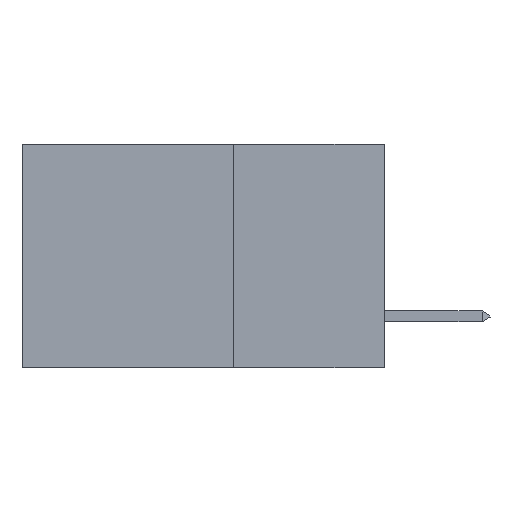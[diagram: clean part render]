
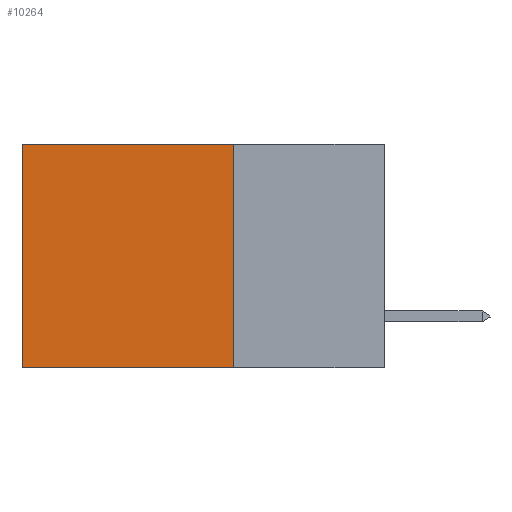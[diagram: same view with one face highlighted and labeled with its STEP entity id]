
A CAD part, left-side view. The second image highlights one B-rep face of the part: STEP entity #10264.
In plain terms, the highlighted planar face has unit normal (-1, 0, 0).
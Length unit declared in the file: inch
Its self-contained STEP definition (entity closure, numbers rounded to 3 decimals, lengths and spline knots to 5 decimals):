
#300 = CARTESIAN_POINT ( 'NONE',  ( 0.2875, 0.25, 0. ) ) ;
#1099 = VERTEX_POINT ( 'NONE', #3515 ) ;
#1140 = LINE ( 'NONE', #6126, #1829 ) ;
#1829 = VECTOR ( 'NONE', #17146, 39.37008 ) ;
#2435 = EDGE_CURVE ( 'NONE', #11167, #4424, #5220, .T. ) ;
#2447 = CARTESIAN_POINT ( 'NONE',  ( 0.2875, 0.25, -0.37 ) ) ;
#3110 = CARTESIAN_POINT ( 'NONE',  ( 0.2875, 0.25, 0. ) ) ;
#3515 = CARTESIAN_POINT ( 'NONE',  ( 0.2875, 0.6, 0. ) ) ;
#3711 = VECTOR ( 'NONE', #9554, 39.37008 ) ;
#4189 = CARTESIAN_POINT ( 'NONE',  ( 0.2875, 0.25, -0.37 ) ) ;
#4190 = VECTOR ( 'NONE', #6963, 39.37008 ) ;
#4424 = VERTEX_POINT ( 'NONE', #2447 ) ;
#4636 = VECTOR ( 'NONE', #16760, 39.37008 ) ;
#5220 = LINE ( 'NONE', #15196, #3711 ) ;
#5274 = FACE_OUTER_BOUND ( 'NONE', #11507, .T. ) ;
#5278 = ORIENTED_EDGE ( 'NONE', *, *, #16095, .F. ) ;
#6126 = CARTESIAN_POINT ( 'NONE',  ( 0.2875, 0.6, 0. ) ) ;
#6963 = DIRECTION ( 'NONE',  ( 0., 1., 0. ) ) ;
#7256 = VERTEX_POINT ( 'NONE', #7313 ) ;
#7297 = DIRECTION ( 'NONE',  ( 0., 0., -1. ) ) ;
#7313 = CARTESIAN_POINT ( 'NONE',  ( 0.2875, 0.6, -0.37 ) ) ;
#8402 = EDGE_CURVE ( 'NONE', #1099, #7256, #1140, .T. ) ;
#9554 = DIRECTION ( 'NONE',  ( 0., 0., -1. ) ) ;
#10019 = ORIENTED_EDGE ( 'NONE', *, *, #2435, .F. ) ;
#10062 = DIRECTION ( 'NONE',  ( 1., 0., 0. ) ) ;
#10264 = ADVANCED_FACE ( 'NONE', ( #5274 ), #11412, .F. ) ;
#11167 = VERTEX_POINT ( 'NONE', #300 ) ;
#11385 = CARTESIAN_POINT ( 'NONE',  ( 0.2875, 0.25, 0. ) ) ;
#11386 = LINE ( 'NONE', #11385, #4190 ) ;
#11412 = PLANE ( 'NONE',  #16078 ) ;
#11507 = EDGE_LOOP ( 'NONE', ( #14045, #5278, #10019, #16907 ) ) ;
#14045 = ORIENTED_EDGE ( 'NONE', *, *, #8402, .T. ) ;
#15196 = CARTESIAN_POINT ( 'NONE',  ( 0.2875, 0.25, 0. ) ) ;
#15967 = LINE ( 'NONE', #4189, #4636 ) ;
#16052 = EDGE_CURVE ( 'NONE', #11167, #1099, #11386, .T. ) ;
#16078 = AXIS2_PLACEMENT_3D ( 'NONE', #3110, #10062, #7297 ) ;
#16095 = EDGE_CURVE ( 'NONE', #4424, #7256, #15967, .T. ) ;
#16760 = DIRECTION ( 'NONE',  ( 0., 1., 0. ) ) ;
#16907 = ORIENTED_EDGE ( 'NONE', *, *, #16052, .T. ) ;
#17146 = DIRECTION ( 'NONE',  ( 0., 0., -1. ) ) ;
